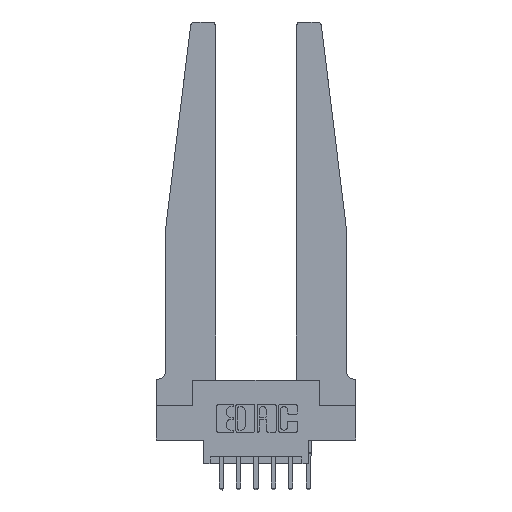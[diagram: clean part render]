
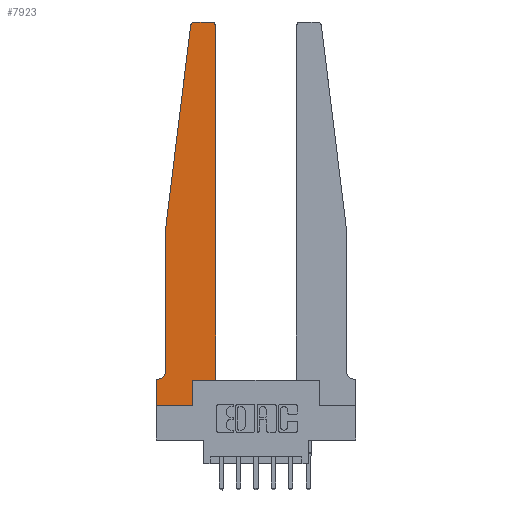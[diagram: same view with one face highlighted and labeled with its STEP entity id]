
A CAD part, top view. The second image highlights one B-rep face of the part: STEP entity #7923.
In plain terms, the highlighted planar face has unit normal (0, 0, 1).
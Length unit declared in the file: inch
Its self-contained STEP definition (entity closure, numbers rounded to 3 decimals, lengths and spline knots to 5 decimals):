
#98 = VECTOR ( 'NONE', #13100, 39.37008 ) ;
#143 = VERTEX_POINT ( 'NONE', #1578 ) ;
#149 = CARTESIAN_POINT ( 'NONE',  ( 0.065, 0.1875, 0.37 ) ) ;
#172 = VERTEX_POINT ( 'NONE', #7005 ) ;
#213 = LINE ( 'NONE', #149, #8026 ) ;
#256 = FACE_OUTER_BOUND ( 'NONE', #7635, .T. ) ;
#313 = LINE ( 'NONE', #2453, #6719 ) ;
#636 = ORIENTED_EDGE ( 'NONE', *, *, #6240, .T. ) ;
#1121 = DIRECTION ( 'NONE',  ( -1., 0., 0. ) ) ;
#1155 = AXIS2_PLACEMENT_3D ( 'NONE', #5053, #5203, #5133 ) ;
#1227 = DIRECTION ( 'NONE',  ( 1., 0., 0. ) ) ;
#1468 = DIRECTION ( 'NONE',  ( 1., 0., 0. ) ) ;
#1578 = CARTESIAN_POINT ( 'NONE',  ( 0.065, 1.25, 0.37 ) ) ;
#1580 = CARTESIAN_POINT ( 'NONE',  ( 0.065, 0.2375, 0.37 ) ) ;
#1805 = VERTEX_POINT ( 'NONE', #5435 ) ;
#1848 = CARTESIAN_POINT ( 'NONE',  ( 0., 0., 0.37 ) ) ;
#2079 = ORIENTED_EDGE ( 'NONE', *, *, #2597, .T. ) ;
#2240 = VERTEX_POINT ( 'NONE', #13632 ) ;
#2315 = ORIENTED_EDGE ( 'NONE', *, *, #6884, .T. ) ;
#2453 = CARTESIAN_POINT ( 'NONE',  ( 0.425, 0.18, 0.37 ) ) ;
#2517 = VERTEX_POINT ( 'NONE', #9447 ) ;
#2573 = DIRECTION ( 'NONE',  ( 0., 1., 0. ) ) ;
#2597 = EDGE_CURVE ( 'NONE', #172, #10479, #313, .T. ) ;
#3148 = EDGE_CURVE ( 'NONE', #9369, #143, #8790, .T. ) ;
#3251 = VERTEX_POINT ( 'NONE', #3680 ) ;
#3267 = ORIENTED_EDGE ( 'NONE', *, *, #3148, .T. ) ;
#3680 = CARTESIAN_POINT ( 'NONE',  ( 0.2605, 0., 0.37 ) ) ;
#3737 = ORIENTED_EDGE ( 'NONE', *, *, #8175, .T. ) ;
#3990 = CIRCLE ( 'NONE', #10005, 0.03 ) ;
#4045 = CARTESIAN_POINT ( 'NONE',  ( 0.425, 0.18, 0.37 ) ) ;
#4130 = EDGE_CURVE ( 'NONE', #143, #9129, #6982, .T. ) ;
#4543 = CARTESIAN_POINT ( 'NONE',  ( 0.015, 0.2375, 0.37 ) ) ;
#5053 = CARTESIAN_POINT ( 'NONE',  ( 0.395, 2.72, 0.37 ) ) ;
#5133 = DIRECTION ( 'NONE',  ( 1., 0., 0. ) ) ;
#5203 = DIRECTION ( 'NONE',  ( 0., 0., 1. ) ) ;
#5232 = ORIENTED_EDGE ( 'NONE', *, *, #12971, .T. ) ;
#5435 = CARTESIAN_POINT ( 'NONE',  ( 0., 0.1875, 0.37 ) ) ;
#5638 = CARTESIAN_POINT ( 'NONE',  ( 0.065, 1.25, 0.37 ) ) ;
#5935 = VECTOR ( 'NONE', #13396, 39.37008 ) ;
#5984 = DIRECTION ( 'NONE',  ( 1., 0., 0. ) ) ;
#6044 = CARTESIAN_POINT ( 'NONE',  ( 0.25, 2.75, 0.37 ) ) ;
#6083 = DIRECTION ( 'NONE',  ( 0., -1., 0. ) ) ;
#6126 = LINE ( 'NONE', #4045, #7078 ) ;
#6240 = EDGE_CURVE ( 'NONE', #1805, #10270, #7137, .T. ) ;
#6264 = ORIENTED_EDGE ( 'NONE', *, *, #10042, .T. ) ;
#6374 = ORIENTED_EDGE ( 'NONE', *, *, #8279, .T. ) ;
#6719 = VECTOR ( 'NONE', #1227, 39.37008 ) ;
#6825 = LINE ( 'NONE', #10181, #10314 ) ;
#6884 = EDGE_CURVE ( 'NONE', #10479, #7435, #6126, .T. ) ;
#6982 = LINE ( 'NONE', #11090, #5935 ) ;
#7005 = CARTESIAN_POINT ( 'NONE',  ( 0.2605, 0.18, 0.37 ) ) ;
#7078 = VECTOR ( 'NONE', #12756, 39.37008 ) ;
#7107 = LINE ( 'NONE', #12173, #10689 ) ;
#7137 = LINE ( 'NONE', #1848, #11503 ) ;
#7381 = LINE ( 'NONE', #6044, #12685 ) ;
#7435 = VERTEX_POINT ( 'NONE', #8774 ) ;
#7517 = DIRECTION ( 'NONE',  ( 0., 0., 1. ) ) ;
#7563 = AXIS2_PLACEMENT_3D ( 'NONE', #4543, #10754, #9907 ) ;
#7635 = EDGE_LOOP ( 'NONE', ( #8683, #9439, #3267, #9518, #3737, #6264, #636, #5232, #6374, #2079, #2315, #8332 ) ) ;
#7817 = CARTESIAN_POINT ( 'NONE',  ( 0.24675, 2.72367, 0.37 ) ) ;
#7923 = ADVANCED_FACE ( 'NONE', ( #256 ), #11934, .T. ) ;
#8004 = VERTEX_POINT ( 'NONE', #9089 ) ;
#8026 = VECTOR ( 'NONE', #1121, 39.37008 ) ;
#8175 = EDGE_CURVE ( 'NONE', #9129, #8004, #11536, .T. ) ;
#8261 = EDGE_CURVE ( 'NONE', #2517, #9369, #3990, .T. ) ;
#8279 = EDGE_CURVE ( 'NONE', #3251, #172, #7107, .T. ) ;
#8332 = ORIENTED_EDGE ( 'NONE', *, *, #10305, .T. ) ;
#8683 = ORIENTED_EDGE ( 'NONE', *, *, #8851, .T. ) ;
#8774 = CARTESIAN_POINT ( 'NONE',  ( 0.425, 2.72, 0.37 ) ) ;
#8790 = LINE ( 'NONE', #5638, #98 ) ;
#8851 = EDGE_CURVE ( 'NONE', #2240, #2517, #7381, .T. ) ;
#9089 = CARTESIAN_POINT ( 'NONE',  ( 0.015, 0.1875, 0.37 ) ) ;
#9129 = VERTEX_POINT ( 'NONE', #1580 ) ;
#9267 = DIRECTION ( 'NONE',  ( 0., 0., 1. ) ) ;
#9369 = VERTEX_POINT ( 'NONE', #7817 ) ;
#9439 = ORIENTED_EDGE ( 'NONE', *, *, #8261, .T. ) ;
#9447 = CARTESIAN_POINT ( 'NONE',  ( 0.27653, 2.75, 0.37 ) ) ;
#9518 = ORIENTED_EDGE ( 'NONE', *, *, #4130, .T. ) ;
#9529 = CARTESIAN_POINT ( 'NONE',  ( 0., 0.1875, 0.37 ) ) ;
#9826 = CIRCLE ( 'NONE', #1155, 0.03 ) ;
#9907 = DIRECTION ( 'NONE',  ( -1., 0., 0. ) ) ;
#10005 = AXIS2_PLACEMENT_3D ( 'NONE', #13315, #9267, #5984 ) ;
#10042 = EDGE_CURVE ( 'NONE', #8004, #1805, #213, .T. ) ;
#10181 = CARTESIAN_POINT ( 'NONE',  ( 0., 0., 0.37 ) ) ;
#10270 = VERTEX_POINT ( 'NONE', #12511 ) ;
#10305 = EDGE_CURVE ( 'NONE', #7435, #2240, #9826, .T. ) ;
#10314 = VECTOR ( 'NONE', #1468, 39.37008 ) ;
#10479 = VERTEX_POINT ( 'NONE', #10642 ) ;
#10642 = CARTESIAN_POINT ( 'NONE',  ( 0.425, 0.18, 0.37 ) ) ;
#10689 = VECTOR ( 'NONE', #2573, 39.37008 ) ;
#10754 = DIRECTION ( 'NONE',  ( 0., 0., -1. ) ) ;
#11090 = CARTESIAN_POINT ( 'NONE',  ( 0.065, 1.25, 0.37 ) ) ;
#11503 = VECTOR ( 'NONE', #6083, 39.37008 ) ;
#11536 = CIRCLE ( 'NONE', #7563, 0.05 ) ;
#11538 = DIRECTION ( 'NONE',  ( -1., 0., 0. ) ) ;
#11669 = DIRECTION ( 'NONE',  ( 1., 0., 0. ) ) ;
#11934 = PLANE ( 'NONE',  #13336 ) ;
#12173 = CARTESIAN_POINT ( 'NONE',  ( 0.2605, 0.18, 0.37 ) ) ;
#12511 = CARTESIAN_POINT ( 'NONE',  ( 0., 0., 0.37 ) ) ;
#12685 = VECTOR ( 'NONE', #11538, 39.37008 ) ;
#12756 = DIRECTION ( 'NONE',  ( 0., 1., 0. ) ) ;
#12971 = EDGE_CURVE ( 'NONE', #10270, #3251, #6825, .T. ) ;
#13100 = DIRECTION ( 'NONE',  ( -0.122, -0.992, 0. ) ) ;
#13315 = CARTESIAN_POINT ( 'NONE',  ( 0.27653, 2.72, 0.37 ) ) ;
#13336 = AXIS2_PLACEMENT_3D ( 'NONE', #9529, #7517, #11669 ) ;
#13396 = DIRECTION ( 'NONE',  ( 0., -1., 0. ) ) ;
#13632 = CARTESIAN_POINT ( 'NONE',  ( 0.395, 2.75, 0.37 ) ) ;
